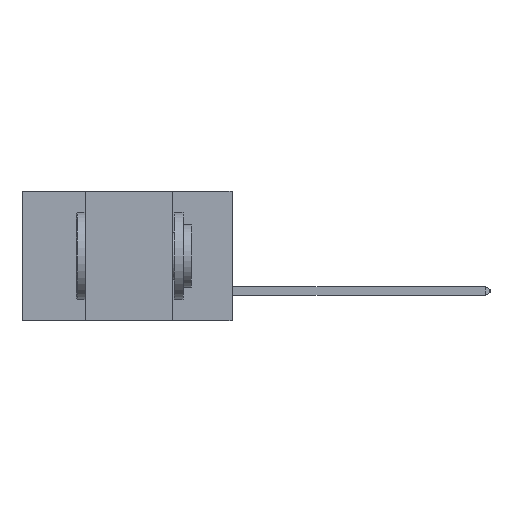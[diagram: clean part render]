
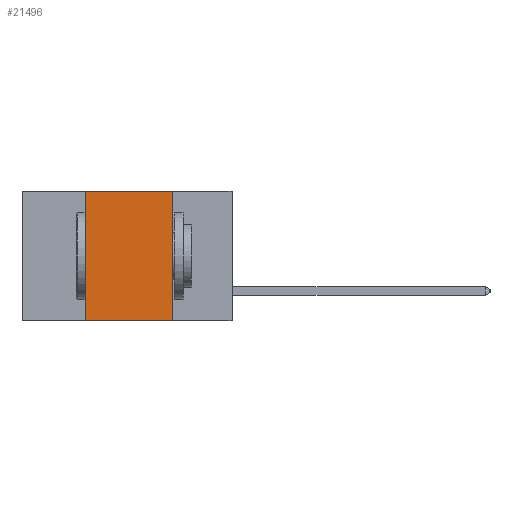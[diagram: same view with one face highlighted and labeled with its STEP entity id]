
A CAD part, left-side view. The second image highlights one B-rep face of the part: STEP entity #21496.
In plain terms, the highlighted planar face has unit normal (-1, 0, 0).
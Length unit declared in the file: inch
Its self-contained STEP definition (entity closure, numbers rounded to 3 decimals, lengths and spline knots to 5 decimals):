
#482 = DIRECTION ( 'NONE',  ( 0., 0., -1. ) ) ;
#1116 = CARTESIAN_POINT ( 'NONE',  ( 0., 0.42, -0.37 ) ) ;
#1180 = VECTOR ( 'NONE', #21974, 39.37008 ) ;
#2146 = FACE_OUTER_BOUND ( 'NONE', #7365, .T. ) ;
#3804 = CARTESIAN_POINT ( 'NONE',  ( 0., 0.6, -0.37 ) ) ;
#7365 = EDGE_LOOP ( 'NONE', ( #22471, #26353, #11837, #13771 ) ) ;
#9320 = CARTESIAN_POINT ( 'NONE',  ( 0., 0.17, 0. ) ) ;
#10590 = CARTESIAN_POINT ( 'NONE',  ( 0., 0.17, -0.37 ) ) ;
#11837 = ORIENTED_EDGE ( 'NONE', *, *, #32271, .F. ) ;
#13771 = ORIENTED_EDGE ( 'NONE', *, *, #34830, .T. ) ;
#14476 = LINE ( 'NONE', #3804, #29937 ) ;
#15875 = CARTESIAN_POINT ( 'NONE',  ( 0., 0.6, 0. ) ) ;
#16075 = AXIS2_PLACEMENT_3D ( 'NONE', #15875, #18995, #482 ) ;
#16643 = VECTOR ( 'NONE', #26142, 39.37008 ) ;
#16745 = VERTEX_POINT ( 'NONE', #36685 ) ;
#16783 = EDGE_CURVE ( 'NONE', #32636, #38656, #36959, .T. ) ;
#18995 = DIRECTION ( 'NONE',  ( 1., 0., 0. ) ) ;
#21491 = EDGE_CURVE ( 'NONE', #16745, #32636, #34017, .T. ) ;
#21496 = ADVANCED_FACE ( 'NONE', ( #2146 ), #34330, .F. ) ;
#21974 = DIRECTION ( 'NONE',  ( 0., -1., 0. ) ) ;
#22471 = ORIENTED_EDGE ( 'NONE', *, *, #16783, .F. ) ;
#23040 = CARTESIAN_POINT ( 'NONE',  ( 0., 0.42, 0. ) ) ;
#24683 = CARTESIAN_POINT ( 'NONE',  ( 0., 0.17, 0. ) ) ;
#24887 = LINE ( 'NONE', #23040, #16643 ) ;
#26142 = DIRECTION ( 'NONE',  ( 0., 0., 1. ) ) ;
#26353 = ORIENTED_EDGE ( 'NONE', *, *, #21491, .F. ) ;
#27765 = DIRECTION ( 'NONE',  ( 0., 0., -1. ) ) ;
#27780 = VERTEX_POINT ( 'NONE', #1116 ) ;
#28163 = CARTESIAN_POINT ( 'NONE',  ( 0., 0.6, 0. ) ) ;
#28542 = DIRECTION ( 'NONE',  ( 0., -1., 0. ) ) ;
#28867 = VECTOR ( 'NONE', #27765, 39.37008 ) ;
#29937 = VECTOR ( 'NONE', #28542, 39.37008 ) ;
#32271 = EDGE_CURVE ( 'NONE', #27780, #16745, #24887, .T. ) ;
#32636 = VERTEX_POINT ( 'NONE', #9320 ) ;
#34017 = LINE ( 'NONE', #28163, #1180 ) ;
#34330 = PLANE ( 'NONE',  #16075 ) ;
#34830 = EDGE_CURVE ( 'NONE', #27780, #38656, #14476, .T. ) ;
#36685 = CARTESIAN_POINT ( 'NONE',  ( 0., 0.42, 0. ) ) ;
#36959 = LINE ( 'NONE', #24683, #28867 ) ;
#38656 = VERTEX_POINT ( 'NONE', #10590 ) ;
